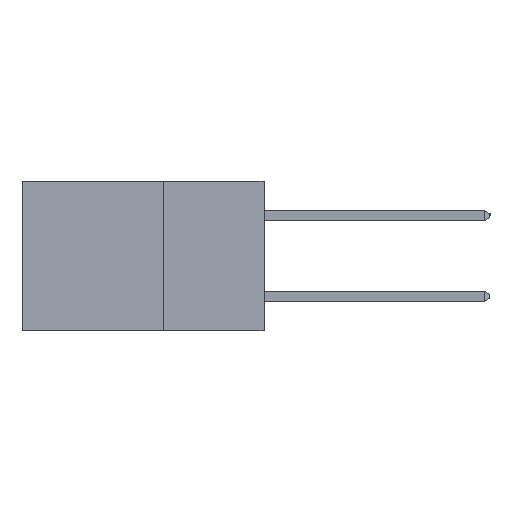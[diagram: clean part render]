
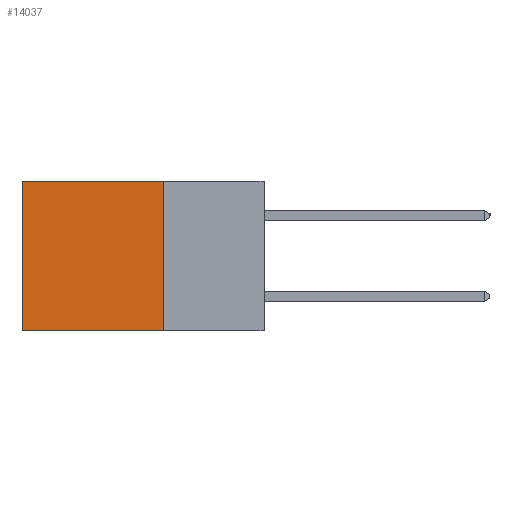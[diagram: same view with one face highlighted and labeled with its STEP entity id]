
A CAD part, left-side view. The second image highlights one B-rep face of the part: STEP entity #14037.
In plain terms, the highlighted planar face has unit normal (-1, 0, 0).
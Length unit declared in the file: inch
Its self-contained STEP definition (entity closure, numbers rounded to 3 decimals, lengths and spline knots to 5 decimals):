
#466 = VERTEX_POINT ( 'NONE', #15859 ) ;
#1655 = DIRECTION ( 'NONE',  ( 1., 0., 0. ) ) ;
#2407 = VERTEX_POINT ( 'NONE', #7561 ) ;
#3875 = CARTESIAN_POINT ( 'NONE',  ( 0.2615, 0.25, -0.37 ) ) ;
#4730 = VECTOR ( 'NONE', #17140, 39.37008 ) ;
#4931 = DIRECTION ( 'NONE',  ( 0., 0., -1. ) ) ;
#5416 = EDGE_LOOP ( 'NONE', ( #12978, #19389, #20278, #13111 ) ) ;
#6716 = EDGE_CURVE ( 'NONE', #2407, #12767, #16821, .T. ) ;
#6725 = LINE ( 'NONE', #10002, #18814 ) ;
#7561 = CARTESIAN_POINT ( 'NONE',  ( 0.2615, 0.25, 0. ) ) ;
#8355 = VECTOR ( 'NONE', #11810, 39.37008 ) ;
#9777 = FACE_OUTER_BOUND ( 'NONE', #5416, .T. ) ;
#10002 = CARTESIAN_POINT ( 'NONE',  ( 0.2615, 0.25, -0.37 ) ) ;
#10604 = CARTESIAN_POINT ( 'NONE',  ( 0.2615, 0.6, 0. ) ) ;
#11108 = VECTOR ( 'NONE', #16870, 39.37008 ) ;
#11358 = CARTESIAN_POINT ( 'NONE',  ( 0.2615, 0.6, -0.37 ) ) ;
#11679 = EDGE_CURVE ( 'NONE', #2407, #20785, #20256, .T. ) ;
#11810 = DIRECTION ( 'NONE',  ( 0., 0., -1. ) ) ;
#12059 = EDGE_CURVE ( 'NONE', #20785, #466, #16743, .T. ) ;
#12767 = VERTEX_POINT ( 'NONE', #3875 ) ;
#12978 = ORIENTED_EDGE ( 'NONE', *, *, #12059, .T. ) ;
#13111 = ORIENTED_EDGE ( 'NONE', *, *, #11679, .T. ) ;
#14037 = ADVANCED_FACE ( 'NONE', ( #9777 ), #19688, .F. ) ;
#14779 = CARTESIAN_POINT ( 'NONE',  ( 0.2615, 0.25, -0.37 ) ) ;
#15859 = CARTESIAN_POINT ( 'NONE',  ( 0.2615, 0.6, -0.37 ) ) ;
#16743 = LINE ( 'NONE', #11358, #8355 ) ;
#16821 = LINE ( 'NONE', #16922, #4730 ) ;
#16870 = DIRECTION ( 'NONE',  ( 0., 1., 0. ) ) ;
#16905 = DIRECTION ( 'NONE',  ( 0., 1., 0. ) ) ;
#16922 = CARTESIAN_POINT ( 'NONE',  ( 0.2615, 0.25, -0.37 ) ) ;
#17140 = DIRECTION ( 'NONE',  ( 0., 0., -1. ) ) ;
#18390 = EDGE_CURVE ( 'NONE', #12767, #466, #6725, .T. ) ;
#18406 = CARTESIAN_POINT ( 'NONE',  ( 0.2615, 0.25, 0. ) ) ;
#18814 = VECTOR ( 'NONE', #16905, 39.37008 ) ;
#18851 = AXIS2_PLACEMENT_3D ( 'NONE', #14779, #1655, #4931 ) ;
#19389 = ORIENTED_EDGE ( 'NONE', *, *, #18390, .F. ) ;
#19688 = PLANE ( 'NONE',  #18851 ) ;
#20256 = LINE ( 'NONE', #18406, #11108 ) ;
#20278 = ORIENTED_EDGE ( 'NONE', *, *, #6716, .F. ) ;
#20785 = VERTEX_POINT ( 'NONE', #10604 ) ;
